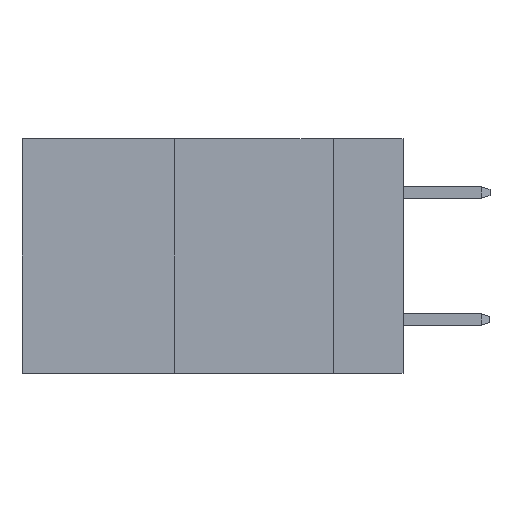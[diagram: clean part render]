
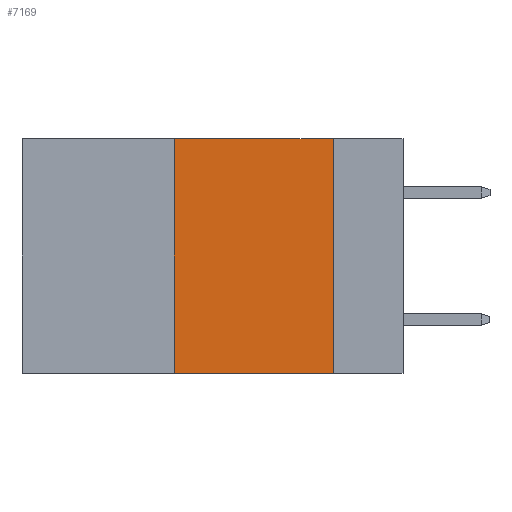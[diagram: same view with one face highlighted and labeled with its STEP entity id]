
A CAD part, left-side view. The second image highlights one B-rep face of the part: STEP entity #7169.
In plain terms, the highlighted planar face has unit normal (-1, 0, 0).
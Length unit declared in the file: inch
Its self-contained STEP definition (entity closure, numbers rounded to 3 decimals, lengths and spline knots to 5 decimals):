
#162 = EDGE_LOOP ( 'NONE', ( #4203, #1346, #8005, #2555 ) ) ;
#181 = VECTOR ( 'NONE', #10086, 39.37008 ) ;
#577 = VECTOR ( 'NONE', #9418, 39.37008 ) ;
#1152 = PLANE ( 'NONE',  #9155 ) ;
#1346 = ORIENTED_EDGE ( 'NONE', *, *, #8964, .F. ) ;
#1719 = CARTESIAN_POINT ( 'NONE',  ( 0., 0.6, 0. ) ) ;
#2555 = ORIENTED_EDGE ( 'NONE', *, *, #10056, .T. ) ;
#2647 = CARTESIAN_POINT ( 'NONE',  ( 0., 0.36, 0. ) ) ;
#2687 = VERTEX_POINT ( 'NONE', #4359 ) ;
#3016 = EDGE_CURVE ( 'NONE', #7285, #6900, #7068, .T. ) ;
#3022 = CARTESIAN_POINT ( 'NONE',  ( 0., 0.36, 0. ) ) ;
#3423 = LINE ( 'NONE', #1719, #5748 ) ;
#3669 = CARTESIAN_POINT ( 'NONE',  ( 0., 0.6, -0.37 ) ) ;
#4203 = ORIENTED_EDGE ( 'NONE', *, *, #8376, .F. ) ;
#4359 = CARTESIAN_POINT ( 'NONE',  ( 0., 0.11, 0. ) ) ;
#4494 = VERTEX_POINT ( 'NONE', #9461 ) ;
#5130 = CARTESIAN_POINT ( 'NONE',  ( 0., 0.36, -0.37 ) ) ;
#5748 = VECTOR ( 'NONE', #9997, 39.37008 ) ;
#6845 = CARTESIAN_POINT ( 'NONE',  ( 0., 0.11, 0. ) ) ;
#6900 = VERTEX_POINT ( 'NONE', #2647 ) ;
#7068 = LINE ( 'NONE', #3022, #9366 ) ;
#7169 = ADVANCED_FACE ( 'NONE', ( #9894 ), #1152, .F. ) ;
#7285 = VERTEX_POINT ( 'NONE', #5130 ) ;
#8005 = ORIENTED_EDGE ( 'NONE', *, *, #3016, .F. ) ;
#8258 = DIRECTION ( 'NONE',  ( 0., 0., -1. ) ) ;
#8376 = EDGE_CURVE ( 'NONE', #2687, #4494, #9186, .T. ) ;
#8463 = CARTESIAN_POINT ( 'NONE',  ( 0., 0.6, 0. ) ) ;
#8763 = DIRECTION ( 'NONE',  ( 0., 0., 1. ) ) ;
#8964 = EDGE_CURVE ( 'NONE', #6900, #2687, #3423, .T. ) ;
#9155 = AXIS2_PLACEMENT_3D ( 'NONE', #8463, #10105, #8258 ) ;
#9186 = LINE ( 'NONE', #6845, #181 ) ;
#9366 = VECTOR ( 'NONE', #8763, 39.37008 ) ;
#9418 = DIRECTION ( 'NONE',  ( 0., -1., 0. ) ) ;
#9460 = LINE ( 'NONE', #3669, #577 ) ;
#9461 = CARTESIAN_POINT ( 'NONE',  ( 0., 0.11, -0.37 ) ) ;
#9894 = FACE_OUTER_BOUND ( 'NONE', #162, .T. ) ;
#9997 = DIRECTION ( 'NONE',  ( 0., -1., 0. ) ) ;
#10056 = EDGE_CURVE ( 'NONE', #7285, #4494, #9460, .T. ) ;
#10086 = DIRECTION ( 'NONE',  ( 0., 0., -1. ) ) ;
#10105 = DIRECTION ( 'NONE',  ( 1., 0., 0. ) ) ;
